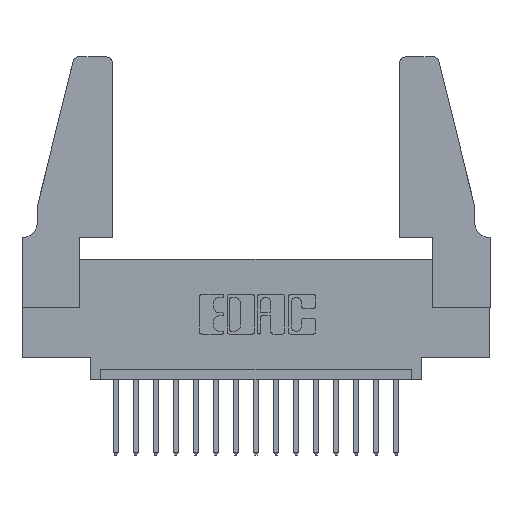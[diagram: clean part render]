
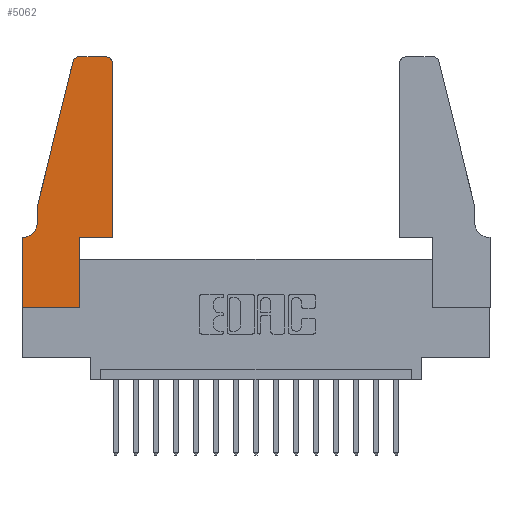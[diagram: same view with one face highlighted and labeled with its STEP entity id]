
A CAD part, top view. The second image highlights one B-rep face of the part: STEP entity #5062.
In plain terms, the highlighted planar face has unit normal (0, 0, 1).
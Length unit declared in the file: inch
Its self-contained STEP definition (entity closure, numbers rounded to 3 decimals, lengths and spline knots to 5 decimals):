
#173 = DIRECTION ( 'NONE',  ( 0., 1., 0. ) ) ;
#450 = CARTESIAN_POINT ( 'NONE',  ( 0., 0.35, 0.37 ) ) ;
#482 = LINE ( 'NONE', #7785, #3809 ) ;
#558 = EDGE_CURVE ( 'NONE', #8261, #5307, #482, .T. ) ;
#589 = DIRECTION ( 'NONE',  ( 1., 0., 0. ) ) ;
#651 = DIRECTION ( 'NONE',  ( 0., 0., 1. ) ) ;
#712 = ORIENTED_EDGE ( 'NONE', *, *, #13703, .T. ) ;
#760 = DIRECTION ( 'NONE',  ( 1., 0., 0. ) ) ;
#811 = CARTESIAN_POINT ( 'NONE',  ( 0., 0.35, 0.37 ) ) ;
#1096 = EDGE_CURVE ( 'NONE', #3043, #5250, #14234, .T. ) ;
#1228 = VERTEX_POINT ( 'NONE', #3066 ) ;
#1231 = CARTESIAN_POINT ( 'NONE',  ( 0.0055, 0.35, 0.37 ) ) ;
#1426 = CARTESIAN_POINT ( 'NONE',  ( 0.2865, 0.35, 0.37 ) ) ;
#1715 = VECTOR ( 'NONE', #12336, 39.37008 ) ;
#1739 = ORIENTED_EDGE ( 'NONE', *, *, #2605, .T. ) ;
#2080 = LINE ( 'NONE', #2182, #15197 ) ;
#2126 = DIRECTION ( 'NONE',  ( -0.239, -0.971, 0. ) ) ;
#2182 = CARTESIAN_POINT ( 'NONE',  ( 0.0755, 0.5, 0.37 ) ) ;
#2492 = DIRECTION ( 'NONE',  ( -1., 0., 0. ) ) ;
#2558 = CARTESIAN_POINT ( 'NONE',  ( 0.0055, 0.42, 0.37 ) ) ;
#2605 = EDGE_CURVE ( 'NONE', #6620, #12739, #3583, .T. ) ;
#2659 = CIRCLE ( 'NONE', #16442, 0.03 ) ;
#2719 = LINE ( 'NONE', #10744, #16240 ) ;
#2972 = ORIENTED_EDGE ( 'NONE', *, *, #16563, .T. ) ;
#3028 = CARTESIAN_POINT ( 'NONE',  ( 0., 0., 0.37 ) ) ;
#3043 = VERTEX_POINT ( 'NONE', #12982 ) ;
#3066 = CARTESIAN_POINT ( 'NONE',  ( 0.25487, 1.22718, 0.37 ) ) ;
#3174 = AXIS2_PLACEMENT_3D ( 'NONE', #8078, #14561, #7915 ) ;
#3322 = CARTESIAN_POINT ( 'NONE',  ( 0.2865, 0.35, 0.37 ) ) ;
#3436 = AXIS2_PLACEMENT_3D ( 'NONE', #2558, #11676, #2492 ) ;
#3524 = EDGE_CURVE ( 'NONE', #9676, #8261, #10437, .T. ) ;
#3583 = LINE ( 'NONE', #3028, #1715 ) ;
#3608 = ORIENTED_EDGE ( 'NONE', *, *, #6608, .T. ) ;
#3809 = VECTOR ( 'NONE', #6384, 39.37008 ) ;
#3836 = ORIENTED_EDGE ( 'NONE', *, *, #13724, .T. ) ;
#4074 = ORIENTED_EDGE ( 'NONE', *, *, #1096, .T. ) ;
#4421 = CARTESIAN_POINT ( 'NONE',  ( 0.284, 1.25, 0.37 ) ) ;
#5062 = ADVANCED_FACE ( 'NONE', ( #12254 ), #7217, .T. ) ;
#5250 = VERTEX_POINT ( 'NONE', #8674 ) ;
#5307 = VERTEX_POINT ( 'NONE', #811 ) ;
#5534 = EDGE_CURVE ( 'NONE', #12739, #9357, #11803, .T. ) ;
#5626 = ORIENTED_EDGE ( 'NONE', *, *, #13036, .T. ) ;
#5802 = VECTOR ( 'NONE', #12754, 39.37008 ) ;
#6218 = VECTOR ( 'NONE', #8505, 39.37008 ) ;
#6384 = DIRECTION ( 'NONE',  ( -1., 0., 0. ) ) ;
#6503 = EDGE_CURVE ( 'NONE', #8998, #9676, #15779, .T. ) ;
#6608 = EDGE_CURVE ( 'NONE', #9357, #15438, #16172, .T. ) ;
#6620 = VERTEX_POINT ( 'NONE', #9227 ) ;
#6634 = VECTOR ( 'NONE', #12097, 39.37008 ) ;
#6647 = EDGE_LOOP ( 'NONE', ( #3836, #16569, #712, #6867, #10371, #12185, #2972, #1739, #12443, #3608, #5626, #4074 ) ) ;
#6867 = ORIENTED_EDGE ( 'NONE', *, *, #6503, .T. ) ;
#7217 = PLANE ( 'NONE',  #17168 ) ;
#7276 = DIRECTION ( 'NONE',  ( 0., 0., 1. ) ) ;
#7785 = CARTESIAN_POINT ( 'NONE',  ( 0.0755, 0.35, 0.37 ) ) ;
#7915 = DIRECTION ( 'NONE',  ( 1., 0., 0. ) ) ;
#8078 = CARTESIAN_POINT ( 'NONE',  ( 0.4205, 1.22, 0.37 ) ) ;
#8098 = CARTESIAN_POINT ( 'NONE',  ( 0., 0., 0.37 ) ) ;
#8261 = VERTEX_POINT ( 'NONE', #1231 ) ;
#8265 = CARTESIAN_POINT ( 'NONE',  ( 0.4505, 0.35, 0.37 ) ) ;
#8505 = DIRECTION ( 'NONE',  ( 0., 1., 0. ) ) ;
#8674 = CARTESIAN_POINT ( 'NONE',  ( 0.4205, 1.25, 0.37 ) ) ;
#8751 = CARTESIAN_POINT ( 'NONE',  ( 0.2605, 1.25, 0.37 ) ) ;
#8998 = VERTEX_POINT ( 'NONE', #9223 ) ;
#9223 = CARTESIAN_POINT ( 'NONE',  ( 0.0755, 0.5, 0.37 ) ) ;
#9227 = CARTESIAN_POINT ( 'NONE',  ( 0., 0., 0.37 ) ) ;
#9357 = VERTEX_POINT ( 'NONE', #1426 ) ;
#9676 = VERTEX_POINT ( 'NONE', #13334 ) ;
#9715 = VECTOR ( 'NONE', #11934, 39.37008 ) ;
#10258 = CARTESIAN_POINT ( 'NONE',  ( 0.2865, 0., 0.37 ) ) ;
#10371 = ORIENTED_EDGE ( 'NONE', *, *, #3524, .T. ) ;
#10437 = CIRCLE ( 'NONE', #3436, 0.07 ) ;
#10576 = CARTESIAN_POINT ( 'NONE',  ( 0.0755, 0.5, 0.37 ) ) ;
#10744 = CARTESIAN_POINT ( 'NONE',  ( 0.4505, 0.35, 0.37 ) ) ;
#11097 = DIRECTION ( 'NONE',  ( 1., 0., 0. ) ) ;
#11676 = DIRECTION ( 'NONE',  ( 0., 0., -1. ) ) ;
#11803 = LINE ( 'NONE', #3322, #6218 ) ;
#11934 = DIRECTION ( 'NONE',  ( 0., -1., 0. ) ) ;
#12097 = DIRECTION ( 'NONE',  ( 0., -1., 0. ) ) ;
#12185 = ORIENTED_EDGE ( 'NONE', *, *, #558, .T. ) ;
#12254 = FACE_OUTER_BOUND ( 'NONE', #6647, .T. ) ;
#12336 = DIRECTION ( 'NONE',  ( 1., 0., 0. ) ) ;
#12443 = ORIENTED_EDGE ( 'NONE', *, *, #5534, .T. ) ;
#12468 = LINE ( 'NONE', #8751, #5802 ) ;
#12628 = CARTESIAN_POINT ( 'NONE',  ( 0.4505, 0.35, 0.37 ) ) ;
#12739 = VERTEX_POINT ( 'NONE', #10258 ) ;
#12754 = DIRECTION ( 'NONE',  ( -1., 0., 0. ) ) ;
#12982 = CARTESIAN_POINT ( 'NONE',  ( 0.4505, 1.22, 0.37 ) ) ;
#13036 = EDGE_CURVE ( 'NONE', #15438, #3043, #2719, .T. ) ;
#13334 = CARTESIAN_POINT ( 'NONE',  ( 0.0755, 0.42, 0.37 ) ) ;
#13703 = EDGE_CURVE ( 'NONE', #1228, #8998, #2080, .T. ) ;
#13724 = EDGE_CURVE ( 'NONE', #5250, #15946, #12468, .T. ) ;
#14234 = CIRCLE ( 'NONE', #3174, 0.03 ) ;
#14561 = DIRECTION ( 'NONE',  ( 0., 0., 1. ) ) ;
#15197 = VECTOR ( 'NONE', #2126, 39.37008 ) ;
#15438 = VERTEX_POINT ( 'NONE', #8265 ) ;
#15779 = LINE ( 'NONE', #10576, #9715 ) ;
#15831 = LINE ( 'NONE', #8098, #6634 ) ;
#15946 = VERTEX_POINT ( 'NONE', #4421 ) ;
#16172 = LINE ( 'NONE', #12628, #17201 ) ;
#16240 = VECTOR ( 'NONE', #173, 39.37008 ) ;
#16369 = CARTESIAN_POINT ( 'NONE',  ( 0.284, 1.22, 0.37 ) ) ;
#16442 = AXIS2_PLACEMENT_3D ( 'NONE', #16369, #651, #589 ) ;
#16563 = EDGE_CURVE ( 'NONE', #5307, #6620, #15831, .T. ) ;
#16569 = ORIENTED_EDGE ( 'NONE', *, *, #16792, .T. ) ;
#16792 = EDGE_CURVE ( 'NONE', #15946, #1228, #2659, .T. ) ;
#17168 = AXIS2_PLACEMENT_3D ( 'NONE', #450, #7276, #11097 ) ;
#17201 = VECTOR ( 'NONE', #760, 39.37008 ) ;
